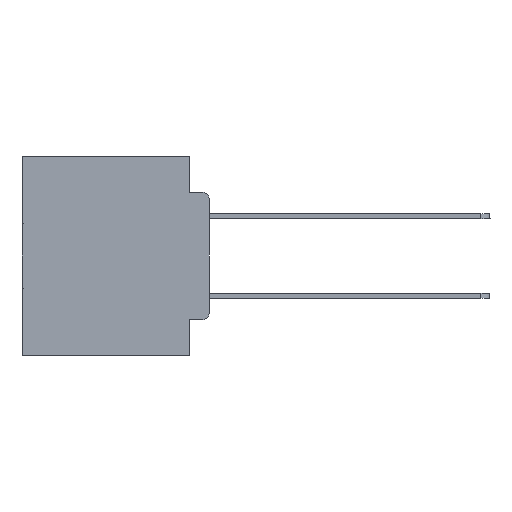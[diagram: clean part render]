
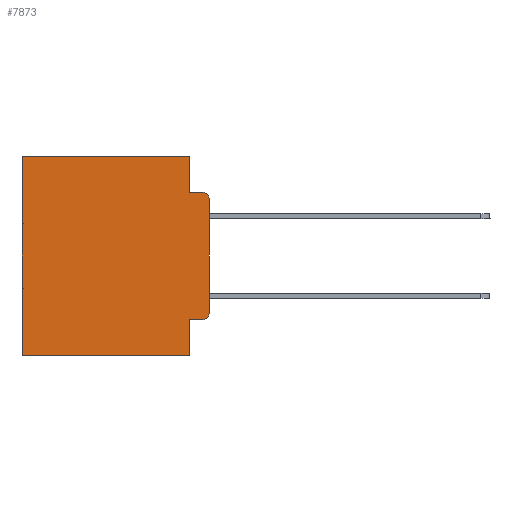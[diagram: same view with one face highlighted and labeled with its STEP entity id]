
A CAD part, left-side view. The second image highlights one B-rep face of the part: STEP entity #7873.
In plain terms, the highlighted planar face has unit normal (-1, 0, 0).
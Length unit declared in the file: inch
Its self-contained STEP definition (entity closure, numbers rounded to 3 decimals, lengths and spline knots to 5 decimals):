
#187 = ORIENTED_EDGE ( 'NONE', *, *, #18495, .F. ) ;
#528 = LINE ( 'NONE', #24044, #25388 ) ;
#1326 = CARTESIAN_POINT ( 'NONE',  ( 0.298, 0.051, -0.5 ) ) ;
#2182 = ORIENTED_EDGE ( 'NONE', *, *, #8246, .T. ) ;
#2264 = CARTESIAN_POINT ( 'NONE',  ( 0.298, 0.051, -0.4115 ) ) ;
#2355 = ORIENTED_EDGE ( 'NONE', *, *, #27119, .F. ) ;
#2737 = ORIENTED_EDGE ( 'NONE', *, *, #24621, .F. ) ;
#3088 = ORIENTED_EDGE ( 'NONE', *, *, #15924, .T. ) ;
#3898 = LINE ( 'NONE', #7161, #30323 ) ;
#4332 = DIRECTION ( 'NONE',  ( 1., 0., 0. ) ) ;
#4605 = LINE ( 'NONE', #13272, #29869 ) ;
#5321 = FACE_OUTER_BOUND ( 'NONE', #16622, .T. ) ;
#5896 = ORIENTED_EDGE ( 'NONE', *, *, #14648, .T. ) ;
#6049 = DIRECTION ( 'NONE',  ( 0., -1., 0. ) ) ;
#6119 = AXIS2_PLACEMENT_3D ( 'NONE', #6310, #8341, #13274 ) ;
#6310 = CARTESIAN_POINT ( 'NONE',  ( 0.298, 0.02, -0.3915 ) ) ;
#6605 = ORIENTED_EDGE ( 'NONE', *, *, #11877, .T. ) ;
#6715 = VERTEX_POINT ( 'NONE', #25363 ) ;
#6759 = DIRECTION ( 'NONE',  ( 0., 0., -1. ) ) ;
#7161 = CARTESIAN_POINT ( 'NONE',  ( 0.298, 0.051, 0. ) ) ;
#7274 = AXIS2_PLACEMENT_3D ( 'NONE', #8171, #27843, #22886 ) ;
#7873 = ADVANCED_FACE ( 'NONE', ( #5321 ), #29039, .F. ) ;
#8013 = DIRECTION ( 'NONE',  ( 0., 1., 0. ) ) ;
#8171 = CARTESIAN_POINT ( 'NONE',  ( 0.298, 0.02, -0.1085 ) ) ;
#8246 = EDGE_CURVE ( 'NONE', #6715, #19351, #24441, .T. ) ;
#8341 = DIRECTION ( 'NONE',  ( -1., 0., 0. ) ) ;
#8448 = CARTESIAN_POINT ( 'NONE',  ( 0.298, 0.051, -0.0885 ) ) ;
#9851 = CIRCLE ( 'NONE', #6119, 0.02 ) ;
#10864 = LINE ( 'NONE', #18665, #23447 ) ;
#11375 = ORIENTED_EDGE ( 'NONE', *, *, #26746, .F. ) ;
#11634 = LINE ( 'NONE', #19043, #20395 ) ;
#11877 = EDGE_CURVE ( 'NONE', #15482, #30681, #17629, .T. ) ;
#12424 = DIRECTION ( 'NONE',  ( 0., 0., -1. ) ) ;
#13151 = VERTEX_POINT ( 'NONE', #30657 ) ;
#13272 = CARTESIAN_POINT ( 'NONE',  ( 0.298, 0., -0.5 ) ) ;
#13274 = DIRECTION ( 'NONE',  ( 0., 0., -1. ) ) ;
#13795 = DIRECTION ( 'NONE',  ( 0., -1., 0. ) ) ;
#13802 = VERTEX_POINT ( 'NONE', #8448 ) ;
#14377 = VERTEX_POINT ( 'NONE', #21758 ) ;
#14593 = CARTESIAN_POINT ( 'NONE',  ( 0.298, 0., 0. ) ) ;
#14648 = EDGE_CURVE ( 'NONE', #14377, #13151, #9851, .T. ) ;
#15482 = VERTEX_POINT ( 'NONE', #28072 ) ;
#15924 = EDGE_CURVE ( 'NONE', #20880, #14377, #10864, .T. ) ;
#16622 = EDGE_LOOP ( 'NONE', ( #2737, #2182, #11375, #2355, #30192, #6605, #187, #18790, #3088, #5896 ) ) ;
#16725 = EDGE_CURVE ( 'NONE', #20880, #25174, #3898, .T. ) ;
#16988 = DIRECTION ( 'NONE',  ( 0., 1., 0. ) ) ;
#17382 = LINE ( 'NONE', #30415, #23486 ) ;
#17629 = LINE ( 'NONE', #31593, #18366 ) ;
#18366 = VECTOR ( 'NONE', #12424, 39.37008 ) ;
#18495 = EDGE_CURVE ( 'NONE', #25174, #30681, #4605, .T. ) ;
#18661 = VECTOR ( 'NONE', #28833, 39.37008 ) ;
#18665 = CARTESIAN_POINT ( 'NONE',  ( 0.298, 0.051, -0.4115 ) ) ;
#18790 = ORIENTED_EDGE ( 'NONE', *, *, #16725, .F. ) ;
#19043 = CARTESIAN_POINT ( 'NONE',  ( 0.298, 0.051, 0. ) ) ;
#19068 = DIRECTION ( 'NONE',  ( 0., 0., -1. ) ) ;
#19351 = VERTEX_POINT ( 'NONE', #26013 ) ;
#20395 = VECTOR ( 'NONE', #31380, 39.37008 ) ;
#20668 = VERTEX_POINT ( 'NONE', #22552 ) ;
#20880 = VERTEX_POINT ( 'NONE', #2264 ) ;
#21758 = CARTESIAN_POINT ( 'NONE',  ( 0.298, 0.02, -0.4115 ) ) ;
#21945 = CARTESIAN_POINT ( 'NONE',  ( 0.298, 0.473, -0.5 ) ) ;
#22552 = CARTESIAN_POINT ( 'NONE',  ( 0.298, 0.051, 0. ) ) ;
#22886 = DIRECTION ( 'NONE',  ( 0., 0., -1. ) ) ;
#23447 = VECTOR ( 'NONE', #13795, 39.37008 ) ;
#23486 = VECTOR ( 'NONE', #6049, 39.37008 ) ;
#24044 = CARTESIAN_POINT ( 'NONE',  ( 0.298, 0., 0. ) ) ;
#24441 = CIRCLE ( 'NONE', #7274, 0.02 ) ;
#24621 = EDGE_CURVE ( 'NONE', #6715, #13151, #27089, .T. ) ;
#25174 = VERTEX_POINT ( 'NONE', #1326 ) ;
#25363 = CARTESIAN_POINT ( 'NONE',  ( 0.298, 0., -0.1085 ) ) ;
#25388 = VECTOR ( 'NONE', #16988, 39.37008 ) ;
#25917 = CARTESIAN_POINT ( 'NONE',  ( 0.298, 0., 0. ) ) ;
#26013 = CARTESIAN_POINT ( 'NONE',  ( 0.298, 0.02, -0.0885 ) ) ;
#26746 = EDGE_CURVE ( 'NONE', #13802, #19351, #17382, .T. ) ;
#27006 = EDGE_CURVE ( 'NONE', #20668, #15482, #528, .T. ) ;
#27089 = LINE ( 'NONE', #25917, #18661 ) ;
#27119 = EDGE_CURVE ( 'NONE', #20668, #13802, #11634, .T. ) ;
#27843 = DIRECTION ( 'NONE',  ( -1., 0., 0. ) ) ;
#28072 = CARTESIAN_POINT ( 'NONE',  ( 0.298, 0.473, 0. ) ) ;
#28833 = DIRECTION ( 'NONE',  ( 0., 0., -1. ) ) ;
#29039 = PLANE ( 'NONE',  #30662 ) ;
#29869 = VECTOR ( 'NONE', #8013, 39.37008 ) ;
#30192 = ORIENTED_EDGE ( 'NONE', *, *, #27006, .T. ) ;
#30323 = VECTOR ( 'NONE', #6759, 39.37008 ) ;
#30415 = CARTESIAN_POINT ( 'NONE',  ( 0.298, 0.051, -0.0885 ) ) ;
#30657 = CARTESIAN_POINT ( 'NONE',  ( 0.298, 0., -0.3915 ) ) ;
#30662 = AXIS2_PLACEMENT_3D ( 'NONE', #14593, #4332, #19068 ) ;
#30681 = VERTEX_POINT ( 'NONE', #21945 ) ;
#31380 = DIRECTION ( 'NONE',  ( 0., 0., -1. ) ) ;
#31593 = CARTESIAN_POINT ( 'NONE',  ( 0.298, 0.473, 0. ) ) ;
